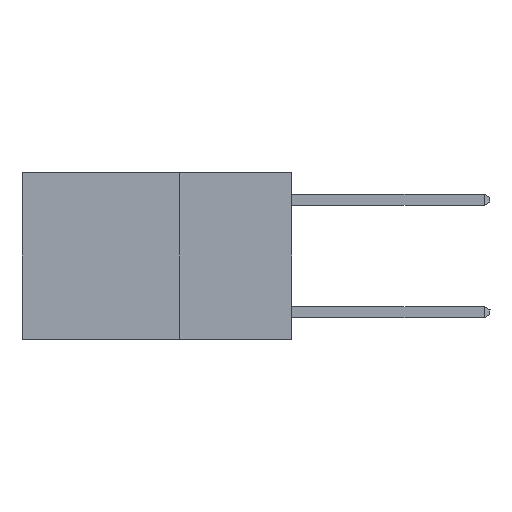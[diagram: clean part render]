
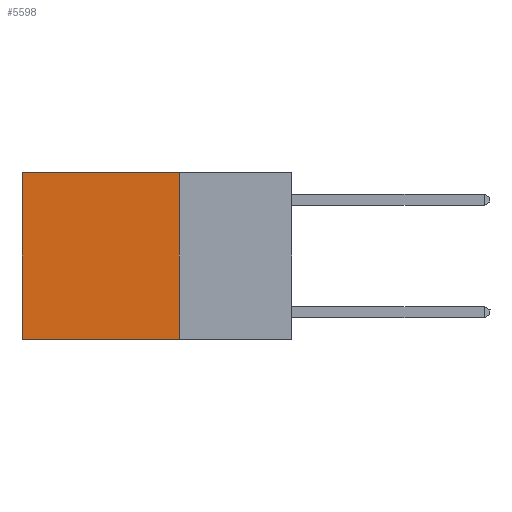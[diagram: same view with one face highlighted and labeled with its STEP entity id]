
A CAD part, left-side view. The second image highlights one B-rep face of the part: STEP entity #5598.
In plain terms, the highlighted planar face has unit normal (-1, 0, 0).
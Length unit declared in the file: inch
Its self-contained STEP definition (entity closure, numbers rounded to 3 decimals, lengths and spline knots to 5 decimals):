
#1525 = CARTESIAN_POINT ( 'NONE',  ( 0.2625, 0.25, 0. ) ) ;
#1829 = VECTOR ( 'NONE', #23548, 39.37008 ) ;
#2122 = EDGE_CURVE ( 'NONE', #15986, #3748, #23430, .T. ) ;
#2502 = FACE_OUTER_BOUND ( 'NONE', #3701, .T. ) ;
#3701 = EDGE_LOOP ( 'NONE', ( #22628, #22960, #23057, #23204 ) ) ;
#3748 = VERTEX_POINT ( 'NONE', #18140 ) ;
#4844 = DIRECTION ( 'NONE',  ( 0., 1., 0. ) ) ;
#5052 = EDGE_CURVE ( 'NONE', #6372, #15986, #14492, .T. ) ;
#5483 = VERTEX_POINT ( 'NONE', #6860 ) ;
#5598 = ADVANCED_FACE ( 'NONE', ( #2502 ), #9616, .F. ) ;
#6372 = VERTEX_POINT ( 'NONE', #1525 ) ;
#6860 = CARTESIAN_POINT ( 'NONE',  ( 0.2625, 0.25, -0.37 ) ) ;
#6985 = CARTESIAN_POINT ( 'NONE',  ( 0.2625, 0.25, 0. ) ) ;
#7012 = DIRECTION ( 'NONE',  ( 0., 1., 0. ) ) ;
#7065 = CARTESIAN_POINT ( 'NONE',  ( 0.2625, 0.6, 0. ) ) ;
#7349 = CARTESIAN_POINT ( 'NONE',  ( 0.2625, 0.25, 0. ) ) ;
#8054 = VECTOR ( 'NONE', #25427, 39.37008 ) ;
#8479 = VECTOR ( 'NONE', #7012, 39.37008 ) ;
#9250 = LINE ( 'NONE', #21485, #1829 ) ;
#9616 = PLANE ( 'NONE',  #11262 ) ;
#10980 = CARTESIAN_POINT ( 'NONE',  ( 0.2625, 0.6, 0. ) ) ;
#11262 = AXIS2_PLACEMENT_3D ( 'NONE', #7349, #11777, #26147 ) ;
#11777 = DIRECTION ( 'NONE',  ( 1., 0., 0. ) ) ;
#13219 = EDGE_CURVE ( 'NONE', #6372, #5483, #9250, .T. ) ;
#14111 = LINE ( 'NONE', #17519, #8479 ) ;
#14492 = LINE ( 'NONE', #6985, #24825 ) ;
#15986 = VERTEX_POINT ( 'NONE', #7065 ) ;
#17519 = CARTESIAN_POINT ( 'NONE',  ( 0.2625, 0.25, -0.37 ) ) ;
#17589 = EDGE_CURVE ( 'NONE', #5483, #3748, #14111, .T. ) ;
#18140 = CARTESIAN_POINT ( 'NONE',  ( 0.2625, 0.6, -0.37 ) ) ;
#21485 = CARTESIAN_POINT ( 'NONE',  ( 0.2625, 0.25, 0. ) ) ;
#22628 = ORIENTED_EDGE ( 'NONE', *, *, #2122, .T. ) ;
#22960 = ORIENTED_EDGE ( 'NONE', *, *, #17589, .F. ) ;
#23057 = ORIENTED_EDGE ( 'NONE', *, *, #13219, .F. ) ;
#23204 = ORIENTED_EDGE ( 'NONE', *, *, #5052, .T. ) ;
#23430 = LINE ( 'NONE', #10980, #8054 ) ;
#23548 = DIRECTION ( 'NONE',  ( 0., 0., -1. ) ) ;
#24825 = VECTOR ( 'NONE', #4844, 39.37008 ) ;
#25427 = DIRECTION ( 'NONE',  ( 0., 0., -1. ) ) ;
#26147 = DIRECTION ( 'NONE',  ( 0., 0., -1. ) ) ;
